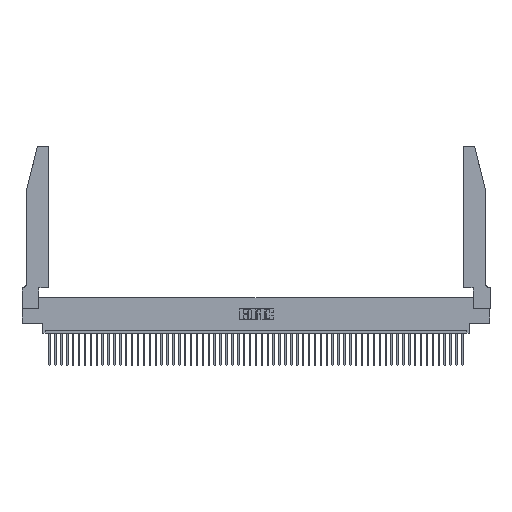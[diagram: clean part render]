
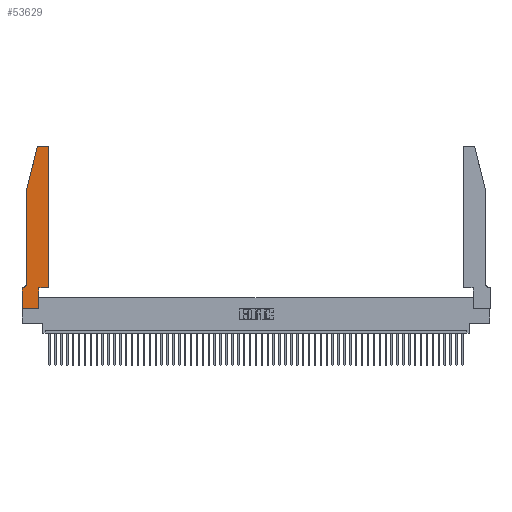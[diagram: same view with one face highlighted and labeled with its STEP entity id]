
A CAD part, top view. The second image highlights one B-rep face of the part: STEP entity #53629.
In plain terms, the highlighted planar face has unit normal (0, 0, 1).
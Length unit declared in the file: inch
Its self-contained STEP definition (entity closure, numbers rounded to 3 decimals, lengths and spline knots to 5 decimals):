
#1542 = LINE ( 'NONE', #30696, #45042 ) ;
#1754 = DIRECTION ( 'NONE',  ( 0., 0., 1. ) ) ;
#2399 = VERTEX_POINT ( 'NONE', #28176 ) ;
#2555 = ORIENTED_EDGE ( 'NONE', *, *, #4995, .T. ) ;
#3805 = VECTOR ( 'NONE', #51735, 39.37008 ) ;
#3891 = DIRECTION ( 'NONE',  ( 1., 0., 0. ) ) ;
#3997 = ORIENTED_EDGE ( 'NONE', *, *, #25730, .T. ) ;
#4258 = CARTESIAN_POINT ( 'NONE',  ( 0.0755, 2., 0.37 ) ) ;
#4995 = EDGE_CURVE ( 'NONE', #39621, #26177, #52018, .T. ) ;
#5305 = VERTEX_POINT ( 'NONE', #41540 ) ;
#5958 = EDGE_CURVE ( 'NONE', #17320, #2399, #10519, .T. ) ;
#6172 = CARTESIAN_POINT ( 'NONE',  ( 0., 0., 0.37 ) ) ;
#6412 = CARTESIAN_POINT ( 'NONE',  ( 0., 0., 0.37 ) ) ;
#7986 = ORIENTED_EDGE ( 'NONE', *, *, #24562, .T. ) ;
#8226 = VECTOR ( 'NONE', #28669, 39.37008 ) ;
#8615 = CARTESIAN_POINT ( 'NONE',  ( 0.0755, 0.35, 0.37 ) ) ;
#8927 = CIRCLE ( 'NONE', #9037, 0.07 ) ;
#9037 = AXIS2_PLACEMENT_3D ( 'NONE', #12094, #11906, #33025 ) ;
#10519 = LINE ( 'NONE', #52298, #27543 ) ;
#10736 = EDGE_CURVE ( 'NONE', #36911, #44163, #14656, .T. ) ;
#11906 = DIRECTION ( 'NONE',  ( 0., 0., -1. ) ) ;
#12094 = CARTESIAN_POINT ( 'NONE',  ( 0.0055, 0.42, 0.37 ) ) ;
#12601 = VERTEX_POINT ( 'NONE', #50995 ) ;
#12822 = CARTESIAN_POINT ( 'NONE',  ( 0., 0.35, 0.37 ) ) ;
#14429 = DIRECTION ( 'NONE',  ( -1., 0., 0. ) ) ;
#14510 = CARTESIAN_POINT ( 'NONE',  ( 0.4205, 2.72, 0.37 ) ) ;
#14656 = CIRCLE ( 'NONE', #42429, 0.03 ) ;
#15329 = CARTESIAN_POINT ( 'NONE',  ( 0.4205, 2.75, 0.37 ) ) ;
#17320 = VERTEX_POINT ( 'NONE', #54169 ) ;
#17681 = DIRECTION ( 'NONE',  ( -0.239, -0.971, 0. ) ) ;
#17899 = CARTESIAN_POINT ( 'NONE',  ( 0.0755, 0.42, 0.37 ) ) ;
#18258 = EDGE_CURVE ( 'NONE', #41252, #36911, #31831, .T. ) ;
#19259 = DIRECTION ( 'NONE',  ( 0., 1., 0. ) ) ;
#19373 = LINE ( 'NONE', #47080, #27188 ) ;
#20943 = DIRECTION ( 'NONE',  ( 0., 0., 1. ) ) ;
#22075 = EDGE_CURVE ( 'NONE', #53562, #42182, #29376, .T. ) ;
#22146 = VERTEX_POINT ( 'NONE', #6172 ) ;
#22167 = AXIS2_PLACEMENT_3D ( 'NONE', #41945, #20943, #50349 ) ;
#22419 = EDGE_CURVE ( 'NONE', #22146, #17320, #28032, .T. ) ;
#22441 = EDGE_CURVE ( 'NONE', #12601, #5305, #41938, .T. ) ;
#23069 = VECTOR ( 'NONE', #36717, 39.37008 ) ;
#23484 = ORIENTED_EDGE ( 'NONE', *, *, #53960, .T. ) ;
#24144 = DIRECTION ( 'NONE',  ( 1., 0., 0. ) ) ;
#24175 = VECTOR ( 'NONE', #14429, 39.37008 ) ;
#24467 = CARTESIAN_POINT ( 'NONE',  ( 0.2605, 2.75, 0.37 ) ) ;
#24562 = EDGE_CURVE ( 'NONE', #26177, #53562, #8927, .T. ) ;
#25053 = ORIENTED_EDGE ( 'NONE', *, *, #5958, .T. ) ;
#25730 = EDGE_CURVE ( 'NONE', #44163, #39621, #19373, .T. ) ;
#26014 = EDGE_CURVE ( 'NONE', #5305, #41252, #42351, .T. ) ;
#26177 = VERTEX_POINT ( 'NONE', #17899 ) ;
#27188 = VECTOR ( 'NONE', #17681, 39.37008 ) ;
#27543 = VECTOR ( 'NONE', #19259, 39.37008 ) ;
#27642 = AXIS2_PLACEMENT_3D ( 'NONE', #14510, #1754, #35399 ) ;
#28032 = LINE ( 'NONE', #6412, #3805 ) ;
#28176 = CARTESIAN_POINT ( 'NONE',  ( 0.2865, 0.35, 0.37 ) ) ;
#28669 = DIRECTION ( 'NONE',  ( -1., 0., 0. ) ) ;
#29376 = LINE ( 'NONE', #8615, #24175 ) ;
#30696 = CARTESIAN_POINT ( 'NONE',  ( 0.4505, 0.35, 0.37 ) ) ;
#31831 = LINE ( 'NONE', #24467, #8226 ) ;
#33025 = DIRECTION ( 'NONE',  ( -1., 0., 0. ) ) ;
#33290 = ORIENTED_EDGE ( 'NONE', *, *, #22419, .T. ) ;
#33751 = EDGE_CURVE ( 'NONE', #2399, #12601, #1542, .T. ) ;
#34438 = CARTESIAN_POINT ( 'NONE',  ( 0.25487, 2.72718, 0.37 ) ) ;
#35116 = LINE ( 'NONE', #36162, #38445 ) ;
#35399 = DIRECTION ( 'NONE',  ( 1., 0., 0. ) ) ;
#35767 = DIRECTION ( 'NONE',  ( 0., 1., 0. ) ) ;
#36162 = CARTESIAN_POINT ( 'NONE',  ( 0., 0., 0.37 ) ) ;
#36717 = DIRECTION ( 'NONE',  ( 0., -1., 0. ) ) ;
#36911 = VERTEX_POINT ( 'NONE', #52686 ) ;
#38438 = ORIENTED_EDGE ( 'NONE', *, *, #18258, .T. ) ;
#38445 = VECTOR ( 'NONE', #45007, 39.37008 ) ;
#39214 = VECTOR ( 'NONE', #35767, 39.37008 ) ;
#39299 = ORIENTED_EDGE ( 'NONE', *, *, #22075, .T. ) ;
#39621 = VERTEX_POINT ( 'NONE', #4258 ) ;
#39829 = FACE_OUTER_BOUND ( 'NONE', #45170, .T. ) ;
#40827 = ORIENTED_EDGE ( 'NONE', *, *, #10736, .T. ) ;
#41252 = VERTEX_POINT ( 'NONE', #15329 ) ;
#41540 = CARTESIAN_POINT ( 'NONE',  ( 0.4505, 2.72, 0.37 ) ) ;
#41938 = LINE ( 'NONE', #44047, #39214 ) ;
#41945 = CARTESIAN_POINT ( 'NONE',  ( 0., 0.35, 0.37 ) ) ;
#42101 = PLANE ( 'NONE',  #22167 ) ;
#42182 = VERTEX_POINT ( 'NONE', #12822 ) ;
#42351 = CIRCLE ( 'NONE', #27642, 0.03 ) ;
#42429 = AXIS2_PLACEMENT_3D ( 'NONE', #54212, #46147, #3891 ) ;
#44047 = CARTESIAN_POINT ( 'NONE',  ( 0.4505, 0.35, 0.37 ) ) ;
#44163 = VERTEX_POINT ( 'NONE', #34438 ) ;
#44413 = ORIENTED_EDGE ( 'NONE', *, *, #22441, .T. ) ;
#45007 = DIRECTION ( 'NONE',  ( 0., -1., 0. ) ) ;
#45042 = VECTOR ( 'NONE', #24144, 39.37008 ) ;
#45170 = EDGE_LOOP ( 'NONE', ( #38438, #40827, #3997, #2555, #7986, #39299, #23484, #33290, #25053, #49210, #44413, #47570 ) ) ;
#46147 = DIRECTION ( 'NONE',  ( 0., 0., 1. ) ) ;
#47080 = CARTESIAN_POINT ( 'NONE',  ( 0.0755, 2., 0.37 ) ) ;
#47570 = ORIENTED_EDGE ( 'NONE', *, *, #26014, .T. ) ;
#48288 = CARTESIAN_POINT ( 'NONE',  ( 0.0755, 2., 0.37 ) ) ;
#49210 = ORIENTED_EDGE ( 'NONE', *, *, #33751, .T. ) ;
#50349 = DIRECTION ( 'NONE',  ( 1., 0., 0. ) ) ;
#50682 = CARTESIAN_POINT ( 'NONE',  ( 0.0055, 0.35, 0.37 ) ) ;
#50995 = CARTESIAN_POINT ( 'NONE',  ( 0.4505, 0.35, 0.37 ) ) ;
#51735 = DIRECTION ( 'NONE',  ( 1., 0., 0. ) ) ;
#52018 = LINE ( 'NONE', #48288, #23069 ) ;
#52298 = CARTESIAN_POINT ( 'NONE',  ( 0.2865, 0.35, 0.37 ) ) ;
#52686 = CARTESIAN_POINT ( 'NONE',  ( 0.284, 2.75, 0.37 ) ) ;
#53562 = VERTEX_POINT ( 'NONE', #50682 ) ;
#53629 = ADVANCED_FACE ( 'NONE', ( #39829 ), #42101, .T. ) ;
#53960 = EDGE_CURVE ( 'NONE', #42182, #22146, #35116, .T. ) ;
#54169 = CARTESIAN_POINT ( 'NONE',  ( 0.2865, 0., 0.37 ) ) ;
#54212 = CARTESIAN_POINT ( 'NONE',  ( 0.284, 2.72, 0.37 ) ) ;
